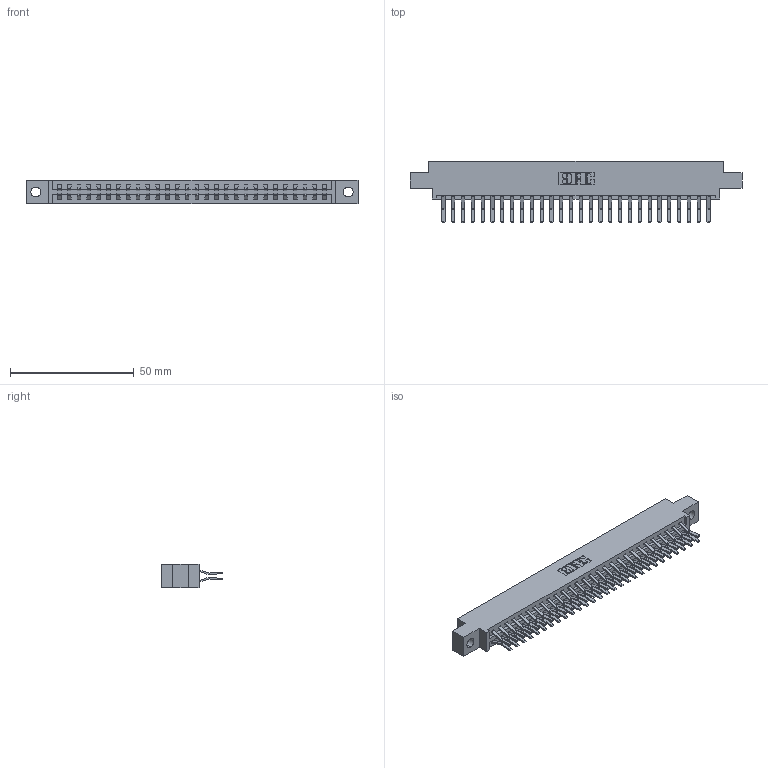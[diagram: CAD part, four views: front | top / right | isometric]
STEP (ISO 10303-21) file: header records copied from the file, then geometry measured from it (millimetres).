
FILE_DESCRIPTION (( 'STEP AP203' ), '1' );
FILE_NAME ('387-056-560-804.STEP', '2018-09-21T00:46:45', ( '' ), ( '' ), 'SwSTEP 2.0', 'SolidWorks 2016', '' );
FILE_SCHEMA (( 'CONFIG_CONTROL_DESIGN' ));
Length unit declared in the file: inch
Products named in the file (3): 337 Part_0.170 Offset - 0.156 Dia-TH; 345-292-001_560 Tail; 387-056-560-804
Assembly tree (57 placements, depth 2):
  387-056-560-804
    337 Part_0.170 Offset - 0.156 Dia-TH
    345-292-001_560 Tail  x56
Bounding box: 133.96 x 24.78 x 9.4 mm (x, y, z)
Volume: 14093.1 mm3; surface area: 16763.8 mm2
Topology: 57 solids, 57 shells, 3254 faces, 9675 edges, 6374 vertices
Faces by surface type: plane 2202, cylinder 1052
Entity records: 23743 total; most frequent: CARTESIAN_POINT 4014, ORIENTED_EDGE 3950, DIRECTION 3443, EDGE_CURVE 1975, LINE 1843, VECTOR 1843, VERTEX_POINT 1314, AXIS2_PLACEMENT_3D 800
